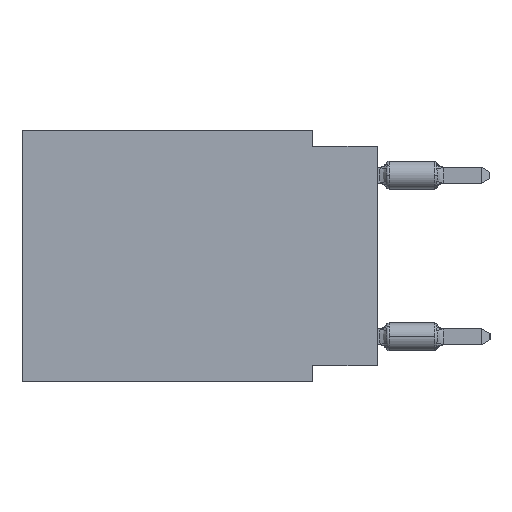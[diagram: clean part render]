
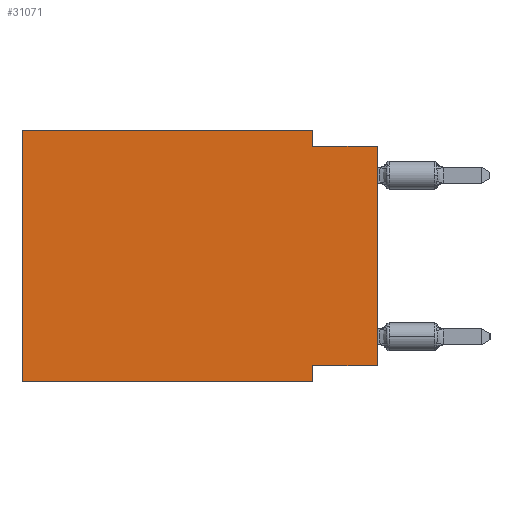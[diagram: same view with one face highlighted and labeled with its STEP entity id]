
A CAD part, left-side view. The second image highlights one B-rep face of the part: STEP entity #31071.
In plain terms, the highlighted planar face has unit normal (-1, 0, 0).
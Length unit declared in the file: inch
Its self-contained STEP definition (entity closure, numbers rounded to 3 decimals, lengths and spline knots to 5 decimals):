
#219 = CARTESIAN_POINT ( 'NONE',  ( 0., 0.55, 0. ) ) ;
#3738 = PLANE ( 'NONE',  #7661 ) ;
#4088 = EDGE_CURVE ( 'NONE', #24628, #44110, #31858, .T. ) ;
#4529 = EDGE_CURVE ( 'NONE', #11960, #34821, #13685, .T. ) ;
#6383 = CARTESIAN_POINT ( 'NONE',  ( 0., 0.55, -0.39 ) ) ;
#6871 = CARTESIAN_POINT ( 'NONE',  ( 0., 0.55, -0.39 ) ) ;
#7027 = VERTEX_POINT ( 'NONE', #34528 ) ;
#7280 = FACE_OUTER_BOUND ( 'NONE', #44842, .T. ) ;
#7661 = AXIS2_PLACEMENT_3D ( 'NONE', #8436, #34147, #11668 ) ;
#8113 = CARTESIAN_POINT ( 'NONE',  ( 0., 0., -0.025 ) ) ;
#8165 = ORIENTED_EDGE ( 'NONE', *, *, #46190, .F. ) ;
#8408 = DIRECTION ( 'NONE',  ( 0., -1., 0. ) ) ;
#8436 = CARTESIAN_POINT ( 'NONE',  ( 0., 0.55, 0. ) ) ;
#9104 = ORIENTED_EDGE ( 'NONE', *, *, #34887, .T. ) ;
#10521 = CARTESIAN_POINT ( 'NONE',  ( 0., 0.55, 0. ) ) ;
#10701 = VECTOR ( 'NONE', #45835, 39.37008 ) ;
#11045 = VERTEX_POINT ( 'NONE', #34807 ) ;
#11668 = DIRECTION ( 'NONE',  ( 0., 0., -1. ) ) ;
#11960 = VERTEX_POINT ( 'NONE', #6383 ) ;
#13685 = LINE ( 'NONE', #219, #10701 ) ;
#16673 = CARTESIAN_POINT ( 'NONE',  ( 0., 0.55, 0. ) ) ;
#19192 = DIRECTION ( 'NONE',  ( 0., 0., -1. ) ) ;
#19482 = CARTESIAN_POINT ( 'NONE',  ( 0., 0.1, 0. ) ) ;
#19570 = DIRECTION ( 'NONE',  ( 0., 0., -1. ) ) ;
#20643 = ORIENTED_EDGE ( 'NONE', *, *, #53988, .T. ) ;
#22807 = CARTESIAN_POINT ( 'NONE',  ( 0., 0.1, -0.39 ) ) ;
#24628 = VERTEX_POINT ( 'NONE', #41459 ) ;
#27095 = EDGE_CURVE ( 'NONE', #30723, #24628, #46755, .T. ) ;
#28325 = DIRECTION ( 'NONE',  ( 0., 0., 1. ) ) ;
#28537 = LINE ( 'NONE', #19482, #46812 ) ;
#28900 = DIRECTION ( 'NONE',  ( 0., 1., 0. ) ) ;
#30036 = VERTEX_POINT ( 'NONE', #41624 ) ;
#30723 = VERTEX_POINT ( 'NONE', #43275 ) ;
#30968 = LINE ( 'NONE', #16673, #50231 ) ;
#31071 = ADVANCED_FACE ( 'NONE', ( #7280 ), #3738, .F. ) ;
#31858 = LINE ( 'NONE', #22807, #40473 ) ;
#32994 = LINE ( 'NONE', #51434, #46104 ) ;
#33242 = ORIENTED_EDGE ( 'NONE', *, *, #36784, .F. ) ;
#33283 = CARTESIAN_POINT ( 'NONE',  ( 0., 0., -0.365 ) ) ;
#34147 = DIRECTION ( 'NONE',  ( 1., 0., 0. ) ) ;
#34528 = CARTESIAN_POINT ( 'NONE',  ( 0., 0.1, 0. ) ) ;
#34807 = CARTESIAN_POINT ( 'NONE',  ( 0., 0., -0.025 ) ) ;
#34821 = VERTEX_POINT ( 'NONE', #10521 ) ;
#34887 = EDGE_CURVE ( 'NONE', #30723, #11045, #32994, .T. ) ;
#36750 = VECTOR ( 'NONE', #40078, 39.37008 ) ;
#36784 = EDGE_CURVE ( 'NONE', #7027, #30036, #28537, .T. ) ;
#39418 = ORIENTED_EDGE ( 'NONE', *, *, #4088, .F. ) ;
#40078 = DIRECTION ( 'NONE',  ( 0., -1., 0. ) ) ;
#40104 = EDGE_CURVE ( 'NONE', #30036, #11045, #52271, .T. ) ;
#40473 = VECTOR ( 'NONE', #19570, 39.37008 ) ;
#41459 = CARTESIAN_POINT ( 'NONE',  ( 0., 0.1, -0.365 ) ) ;
#41471 = ORIENTED_EDGE ( 'NONE', *, *, #4529, .F. ) ;
#41624 = CARTESIAN_POINT ( 'NONE',  ( 0., 0.1, -0.025 ) ) ;
#42570 = ORIENTED_EDGE ( 'NONE', *, *, #40104, .F. ) ;
#43275 = CARTESIAN_POINT ( 'NONE',  ( 0., 0., -0.365 ) ) ;
#43675 = CARTESIAN_POINT ( 'NONE',  ( 0., 0.1, -0.39 ) ) ;
#43840 = VECTOR ( 'NONE', #28900, 39.37008 ) ;
#44110 = VERTEX_POINT ( 'NONE', #43675 ) ;
#44842 = EDGE_LOOP ( 'NONE', ( #9104, #42570, #33242, #8165, #41471, #20643, #39418, #49258 ) ) ;
#45835 = DIRECTION ( 'NONE',  ( 0., 0., 1. ) ) ;
#46104 = VECTOR ( 'NONE', #28325, 39.37008 ) ;
#46190 = EDGE_CURVE ( 'NONE', #34821, #7027, #30968, .T. ) ;
#46755 = LINE ( 'NONE', #33283, #43840 ) ;
#46812 = VECTOR ( 'NONE', #19192, 39.37008 ) ;
#47094 = VECTOR ( 'NONE', #8408, 39.37008 ) ;
#48252 = DIRECTION ( 'NONE',  ( 0., -1., 0. ) ) ;
#49258 = ORIENTED_EDGE ( 'NONE', *, *, #27095, .F. ) ;
#50231 = VECTOR ( 'NONE', #48252, 39.37008 ) ;
#51434 = CARTESIAN_POINT ( 'NONE',  ( 0., 0., 0. ) ) ;
#52271 = LINE ( 'NONE', #8113, #47094 ) ;
#53267 = LINE ( 'NONE', #6871, #36750 ) ;
#53988 = EDGE_CURVE ( 'NONE', #11960, #44110, #53267, .T. ) ;
